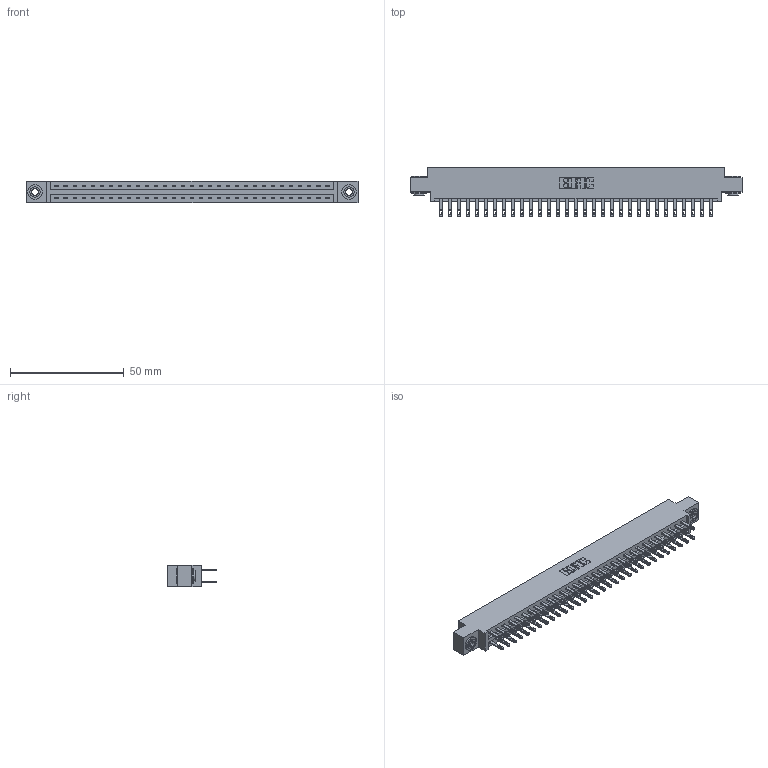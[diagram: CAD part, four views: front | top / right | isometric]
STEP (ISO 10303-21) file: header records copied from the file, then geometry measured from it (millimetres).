
FILE_DESCRIPTION (( 'STEP AP203' ), '1' );
FILE_NAME ('337-062-500-803.STEP', '2018-08-10T09:35:21', ( '' ), ( '' ), 'SwSTEP 2.0', 'SolidWorks 2016', '' );
FILE_SCHEMA (( 'CONFIG_CONTROL_DESIGN' ));
Length unit declared in the file: inch
Products named in the file (4): 345-292-001_345-293-100; 337 Part_0.170 Offset - 0.156 Dia-TH; 345-250-002_345-250-002-102; 337-062-500-803
Assembly tree (65 placements, depth 2):
  337-062-500-803
    337 Part_0.170 Offset - 0.156 Dia-TH
    345-292-001_345-293-100  x62
    345-250-002_345-250-002-102  x2
Bounding box: 145.85 x 21.85 x 9.4 mm (x, y, z)
Volume: 15315.4 mm3; surface area: 18227.4 mm2
Topology: 65 solids, 65 shells, 3256 faces, 9885 edges, 6586 vertices
Faces by surface type: plane 2068, cylinder 1180, cone 8
Entity records: 26170 total; most frequent: CARTESIAN_POINT 4393, ORIENTED_EDGE 4322, DIRECTION 3791, EDGE_CURVE 2161, LINE 2005, VECTOR 2005, VERTEX_POINT 1438, AXIS2_PLACEMENT_3D 893
